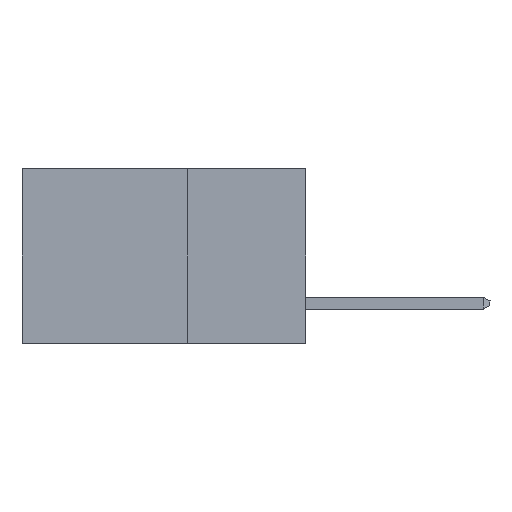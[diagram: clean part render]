
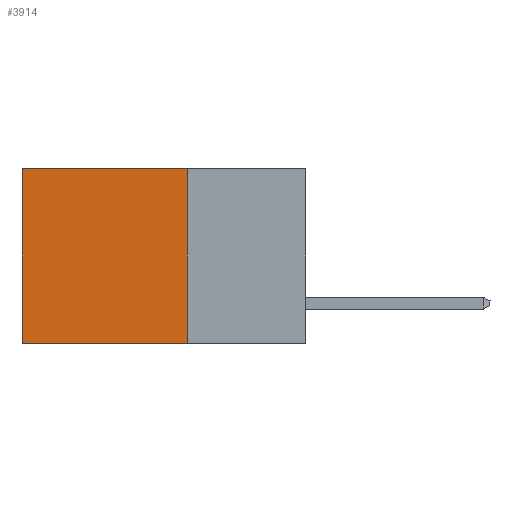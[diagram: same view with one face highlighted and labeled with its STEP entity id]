
A CAD part, left-side view. The second image highlights one B-rep face of the part: STEP entity #3914.
In plain terms, the highlighted planar face has unit normal (-1, 0, 0).
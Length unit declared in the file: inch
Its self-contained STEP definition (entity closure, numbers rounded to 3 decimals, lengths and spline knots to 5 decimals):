
#258 = CARTESIAN_POINT ( 'NONE',  ( 0.298, 0.25, -0.37 ) ) ;
#377 = EDGE_LOOP ( 'NONE', ( #2788, #3505, #6729, #3948 ) ) ;
#1333 = LINE ( 'NONE', #10200, #6032 ) ;
#2323 = VERTEX_POINT ( 'NONE', #5167 ) ;
#2788 = ORIENTED_EDGE ( 'NONE', *, *, #7432, .T. ) ;
#3076 = EDGE_CURVE ( 'NONE', #2323, #10594, #9128, .T. ) ;
#3140 = DIRECTION ( 'NONE',  ( 0., 0., -1. ) ) ;
#3238 = CARTESIAN_POINT ( 'NONE',  ( 0.298, 0.25, -0.37 ) ) ;
#3505 = ORIENTED_EDGE ( 'NONE', *, *, #10295, .F. ) ;
#3540 = VERTEX_POINT ( 'NONE', #4653 ) ;
#3808 = DIRECTION ( 'NONE',  ( 1., 0., 0. ) ) ;
#3914 = ADVANCED_FACE ( 'NONE', ( #9251 ), #9482, .F. ) ;
#3948 = ORIENTED_EDGE ( 'NONE', *, *, #7802, .T. ) ;
#4173 = CARTESIAN_POINT ( 'NONE',  ( 0.298, 0.25, 0. ) ) ;
#4473 = DIRECTION ( 'NONE',  ( 0., 1., 0. ) ) ;
#4653 = CARTESIAN_POINT ( 'NONE',  ( 0.298, 0.6, 0. ) ) ;
#5013 = AXIS2_PLACEMENT_3D ( 'NONE', #7508, #3808, #10431 ) ;
#5167 = CARTESIAN_POINT ( 'NONE',  ( 0.298, 0.25, 0. ) ) ;
#5876 = LINE ( 'NONE', #10939, #11036 ) ;
#6032 = VECTOR ( 'NONE', #8326, 39.37008 ) ;
#6312 = VECTOR ( 'NONE', #3140, 39.37008 ) ;
#6729 = ORIENTED_EDGE ( 'NONE', *, *, #3076, .F. ) ;
#6888 = CARTESIAN_POINT ( 'NONE',  ( 0.298, 0.6, -0.37 ) ) ;
#7432 = EDGE_CURVE ( 'NONE', #3540, #8682, #1333, .T. ) ;
#7508 = CARTESIAN_POINT ( 'NONE',  ( 0.298, 0.25, 0. ) ) ;
#7590 = VECTOR ( 'NONE', #11531, 39.37008 ) ;
#7802 = EDGE_CURVE ( 'NONE', #2323, #3540, #5876, .T. ) ;
#7875 = LINE ( 'NONE', #3238, #7590 ) ;
#8326 = DIRECTION ( 'NONE',  ( 0., 0., -1. ) ) ;
#8682 = VERTEX_POINT ( 'NONE', #6888 ) ;
#9128 = LINE ( 'NONE', #4173, #6312 ) ;
#9251 = FACE_OUTER_BOUND ( 'NONE', #377, .T. ) ;
#9482 = PLANE ( 'NONE',  #5013 ) ;
#10200 = CARTESIAN_POINT ( 'NONE',  ( 0.298, 0.6, 0. ) ) ;
#10295 = EDGE_CURVE ( 'NONE', #10594, #8682, #7875, .T. ) ;
#10431 = DIRECTION ( 'NONE',  ( 0., 0., -1. ) ) ;
#10594 = VERTEX_POINT ( 'NONE', #258 ) ;
#10939 = CARTESIAN_POINT ( 'NONE',  ( 0.298, 0.25, 0. ) ) ;
#11036 = VECTOR ( 'NONE', #4473, 39.37008 ) ;
#11531 = DIRECTION ( 'NONE',  ( 0., 1., 0. ) ) ;
